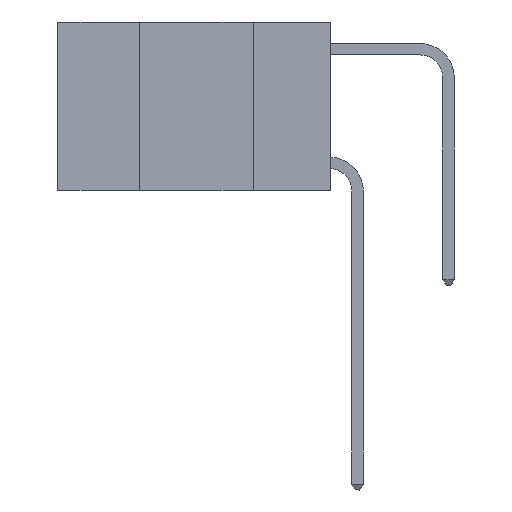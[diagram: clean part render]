
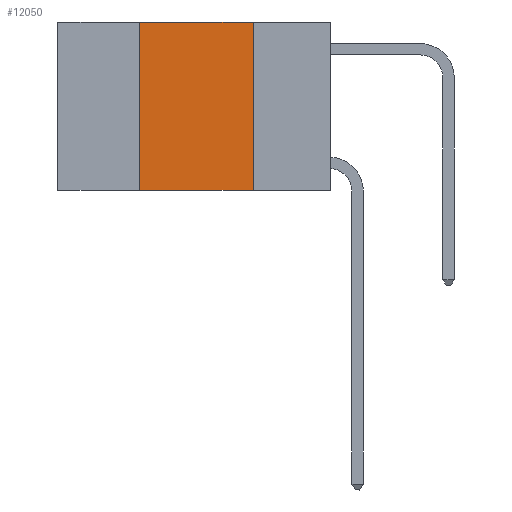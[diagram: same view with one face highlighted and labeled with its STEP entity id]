
A CAD part, left-side view. The second image highlights one B-rep face of the part: STEP entity #12050.
In plain terms, the highlighted planar face has unit normal (-1, 0, 0).
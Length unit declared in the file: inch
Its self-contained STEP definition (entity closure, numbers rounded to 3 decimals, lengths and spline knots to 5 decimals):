
#821 = VECTOR ( 'NONE', #11288, 39.37008 ) ;
#2836 = CARTESIAN_POINT ( 'NONE',  ( 0., 0.17, 0. ) ) ;
#2934 = PLANE ( 'NONE',  #20726 ) ;
#3569 = EDGE_CURVE ( 'NONE', #17048, #4179, #16086, .T. ) ;
#3705 = EDGE_CURVE ( 'NONE', #9103, #20402, #18444, .T. ) ;
#4006 = CARTESIAN_POINT ( 'NONE',  ( 0., 0.42, 0. ) ) ;
#4179 = VERTEX_POINT ( 'NONE', #4006 ) ;
#6965 = VECTOR ( 'NONE', #14366, 39.37008 ) ;
#7761 = VECTOR ( 'NONE', #15644, 39.37008 ) ;
#8109 = DIRECTION ( 'NONE',  ( 1., 0., 0. ) ) ;
#9103 = VERTEX_POINT ( 'NONE', #2836 ) ;
#9202 = CARTESIAN_POINT ( 'NONE',  ( 0., 0.42, 0. ) ) ;
#9422 = ORIENTED_EDGE ( 'NONE', *, *, #3569, .F. ) ;
#10711 = DIRECTION ( 'NONE',  ( 0., -1., 0. ) ) ;
#11288 = DIRECTION ( 'NONE',  ( 0., 0., -1. ) ) ;
#12050 = ADVANCED_FACE ( 'NONE', ( #17793 ), #2934, .F. ) ;
#13006 = CARTESIAN_POINT ( 'NONE',  ( 0., 0.17, 0. ) ) ;
#13484 = EDGE_LOOP ( 'NONE', ( #16909, #21937, #9422, #19560 ) ) ;
#13903 = CARTESIAN_POINT ( 'NONE',  ( 0., 0.6, -0.37 ) ) ;
#14366 = DIRECTION ( 'NONE',  ( 0., 0., 1. ) ) ;
#15644 = DIRECTION ( 'NONE',  ( 0., -1., 0. ) ) ;
#16086 = LINE ( 'NONE', #9202, #6965 ) ;
#16909 = ORIENTED_EDGE ( 'NONE', *, *, #3705, .F. ) ;
#17048 = VERTEX_POINT ( 'NONE', #22030 ) ;
#17257 = EDGE_CURVE ( 'NONE', #4179, #9103, #22075, .T. ) ;
#17560 = VECTOR ( 'NONE', #10711, 39.37008 ) ;
#17793 = FACE_OUTER_BOUND ( 'NONE', #13484, .T. ) ;
#18299 = CARTESIAN_POINT ( 'NONE',  ( 0., 0.6, 0. ) ) ;
#18444 = LINE ( 'NONE', #13006, #821 ) ;
#19560 = ORIENTED_EDGE ( 'NONE', *, *, #20138, .T. ) ;
#20016 = DIRECTION ( 'NONE',  ( 0., 0., -1. ) ) ;
#20138 = EDGE_CURVE ( 'NONE', #17048, #20402, #20806, .T. ) ;
#20402 = VERTEX_POINT ( 'NONE', #21344 ) ;
#20726 = AXIS2_PLACEMENT_3D ( 'NONE', #18299, #8109, #20016 ) ;
#20806 = LINE ( 'NONE', #13903, #7761 ) ;
#20832 = CARTESIAN_POINT ( 'NONE',  ( 0., 0.6, 0. ) ) ;
#21344 = CARTESIAN_POINT ( 'NONE',  ( 0., 0.17, -0.37 ) ) ;
#21937 = ORIENTED_EDGE ( 'NONE', *, *, #17257, .F. ) ;
#22030 = CARTESIAN_POINT ( 'NONE',  ( 0., 0.42, -0.37 ) ) ;
#22075 = LINE ( 'NONE', #20832, #17560 ) ;
